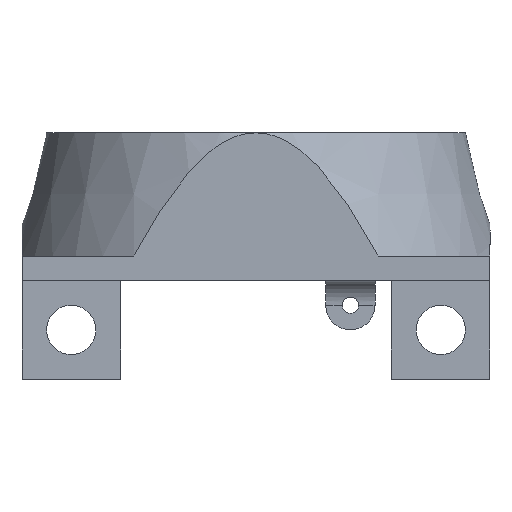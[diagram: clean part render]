
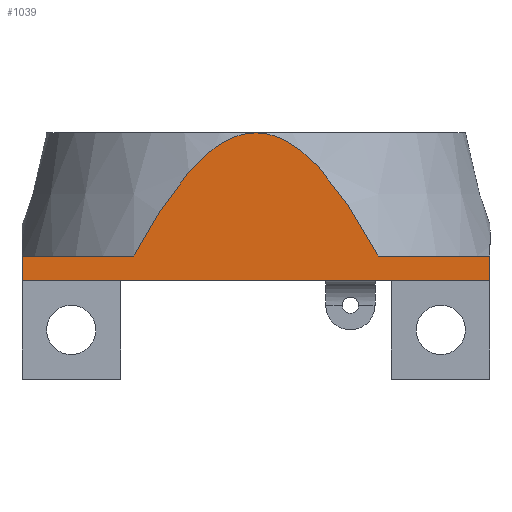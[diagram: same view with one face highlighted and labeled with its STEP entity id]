
A CAD part, left-side view. The second image highlights one B-rep face of the part: STEP entity #1039.
In plain terms, the highlighted planar face has unit normal (-1, 0, 0).
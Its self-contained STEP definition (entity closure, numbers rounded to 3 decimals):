
#65 = CARTESIAN_POINT ( 'NONE',  ( -24.047, 32.051, 2.538 ) ) ;
#81 = EDGE_CURVE ( 'NONE', #1986, #2008, #721, .T. ) ;
#107 = EDGE_CURVE ( 'NONE', #2039, #1986, #688, .T. ) ;
#151 = B_SPLINE_CURVE_WITH_KNOTS ( 'NONE', 3,
 ( #1533, #887, #882, #1527, #1524, #1520, #1516, #1514, #1508, #1505, #1500, #1493, #1483, #1474, #1468, #1466, #1463, #1462, #1455, #1453, #2058, #2047 ),
 .UNSPECIFIED., .F., .F.,
 ( 4, 2, 2, 2, 2, 2, 2, 2, 2, 2, 4 ),
 ( 0., 0.007, 0.01, 0.014, 0.017, 0.019, 0.021, 0.022, 0.024, 0.026, 0.027 ),
 .UNSPECIFIED. ) ;
#364 = DIRECTION ( 'NONE',  ( 0., -1., 0. ) ) ;
#367 = DIRECTION ( 'NONE',  ( 0., 0., -1. ) ) ;
#370 = CARTESIAN_POINT ( 'NONE',  ( -24.047, -0.893, 6.288 ) ) ;
#374 = CARTESIAN_POINT ( 'NONE',  ( -24.047, -39.199, 25.038 ) ) ;
#476 = CARTESIAN_POINT ( 'NONE',  ( -24.047, -39.199, 2.538 ) ) ;
#583 = CARTESIAN_POINT ( 'NONE',  ( -24.047, 32.051, 6.288 ) ) ;
#591 = CARTESIAN_POINT ( 'NONE',  ( -24.047, 15.015, 6.288 ) ) ;
#593 = CARTESIAN_POINT ( 'NONE',  ( -24.047, 13.938, 8.312 ) ) ;
#595 = CARTESIAN_POINT ( 'NONE',  ( -24.047, 12.81, 10.307 ) ) ;
#598 = CARTESIAN_POINT ( 'NONE',  ( -24.047, 10.991, 13.224 ) ) ;
#600 = CARTESIAN_POINT ( 'NONE',  ( -24.047, 10.363, 14.185 ) ) ;
#608 = CARTESIAN_POINT ( 'NONE',  ( -24.047, 9.056, 16.061 ) ) ;
#614 = CARTESIAN_POINT ( 'NONE',  ( -24.047, 8.377, 16.978 ) ) ;
#615 = CARTESIAN_POINT ( 'NONE',  ( -24.047, 6.947, 18.751 ) ) ;
#619 = CARTESIAN_POINT ( 'NONE',  ( -24.047, 6.198, 19.608 ) ) ;
#620 = CARTESIAN_POINT ( 'NONE',  ( -24.047, 4.993, 20.825 ) ) ;
#622 = CARTESIAN_POINT ( 'NONE',  ( -24.047, 4.578, 21.22 ) ) ;
#623 = CARTESIAN_POINT ( 'NONE',  ( -24.047, 3.713, 21.98 ) ) ;
#625 = CARTESIAN_POINT ( 'NONE',  ( -24.047, 3.262, 22.346 ) ) ;
#629 = CARTESIAN_POINT ( 'NONE',  ( -24.047, 1.868, 23.365 ) ) ;
#633 = CARTESIAN_POINT ( 'NONE',  ( -24.047, 0.881, 23.949 ) ) ;
#637 = CARTESIAN_POINT ( 'NONE',  ( -24.047, -1.284, 24.799 ) ) ;
#644 = CARTESIAN_POINT ( 'NONE',  ( -24.047, -3.574, 25.038 ) ) ;
#656 = CARTESIAN_POINT ( 'NONE',  ( -24.047, -2.406, 25.038 ) ) ;
#688 = LINE ( 'NONE', #1654, #696 ) ;
#694 = VECTOR ( 'NONE', #367, 1000. ) ;
#696 = VECTOR ( 'NONE', #1174, 1000. ) ;
#703 = VECTOR ( 'NONE', #364, 1000. ) ;
#710 = VECTOR ( 'NONE', #1718, 1000. ) ;
#714 = LINE ( 'NONE', #370, #703 ) ;
#721 = LINE ( 'NONE', #65, #710 ) ;
#743 = LINE ( 'NONE', #374, #694 ) ;
#747 = CARTESIAN_POINT ( 'NONE',  ( -24.047, 32.051, 2.538 ) ) ;
#825 = CARTESIAN_POINT ( 'NONE',  ( -24.047, 15.015, 6.288 ) ) ;
#849 = EDGE_CURVE ( 'NONE', #2095, #2044, #151, .T. ) ;
#882 = CARTESIAN_POINT ( 'NONE',  ( -24.047, -19.958, 10.305 ) ) ;
#887 = CARTESIAN_POINT ( 'NONE',  ( -24.047, -21.085, 8.312 ) ) ;
#1039 = ADVANCED_FACE ( 'NONE', ( #1063 ), #1399, .F. ) ;
#1063 = FACE_OUTER_BOUND ( 'NONE', #1076, .T. ) ;
#1068 = EDGE_CURVE ( 'NONE', #2095, #2137, #1089, .T. ) ;
#1076 = EDGE_LOOP ( 'NONE', ( #1779, #1772, #1704, #2197, #2210, #1501, #1831 ) ) ;
#1083 = VECTOR ( 'NONE', #1118, 1000. ) ;
#1089 = LINE ( 'NONE', #1121, #1083 ) ;
#1118 = DIRECTION ( 'NONE',  ( 0., -1., 0. ) ) ;
#1121 = CARTESIAN_POINT ( 'NONE',  ( -24.047, -0.893, 6.288 ) ) ;
#1146 = DIRECTION ( 'NONE',  ( 0., 0., -1. ) ) ;
#1149 = DIRECTION ( 'NONE',  ( 1., 0., 0. ) ) ;
#1152 = CARTESIAN_POINT ( 'NONE',  ( -24.047, 32.051, 25.038 ) ) ;
#1174 = DIRECTION ( 'NONE',  ( 0., 0., -1. ) ) ;
#1316 = EDGE_CURVE ( 'NONE', #2044, #2071, #2063, .T. ) ;
#1399 = PLANE ( 'NONE',  #1947 ) ;
#1436 = EDGE_CURVE ( 'NONE', #2137, #2008, #743, .T. ) ;
#1453 = CARTESIAN_POINT ( 'NONE',  ( -24.047, -4.733, 24.978 ) ) ;
#1455 = CARTESIAN_POINT ( 'NONE',  ( -24.047, -5.857, 24.751 ) ) ;
#1458 = EDGE_CURVE ( 'NONE', #2039, #2071, #714, .T. ) ;
#1462 = CARTESIAN_POINT ( 'NONE',  ( -24.047, -6.404, 24.586 ) ) ;
#1463 = CARTESIAN_POINT ( 'NONE',  ( -24.047, -7.473, 24.167 ) ) ;
#1466 = CARTESIAN_POINT ( 'NONE',  ( -24.047, -7.996, 23.913 ) ) ;
#1468 = CARTESIAN_POINT ( 'NONE',  ( -24.047, -8.991, 23.346 ) ) ;
#1474 = CARTESIAN_POINT ( 'NONE',  ( -24.047, -9.469, 23.032 ) ) ;
#1483 = CARTESIAN_POINT ( 'NONE',  ( -24.047, -10.393, 22.358 ) ) ;
#1493 = CARTESIAN_POINT ( 'NONE',  ( -24.047, -10.839, 21.997 ) ) ;
#1500 = CARTESIAN_POINT ( 'NONE',  ( -24.047, -11.705, 21.238 ) ) ;
#1501 = ORIENTED_EDGE ( 'NONE', *, *, #1436, .F. ) ;
#1505 = CARTESIAN_POINT ( 'NONE',  ( -24.047, -12.121, 20.843 ) ) ;
#1508 = CARTESIAN_POINT ( 'NONE',  ( -24.047, -13.33, 19.624 ) ) ;
#1514 = CARTESIAN_POINT ( 'NONE',  ( -24.047, -14.084, 18.763 ) ) ;
#1516 = CARTESIAN_POINT ( 'NONE',  ( -24.047, -15.523, 16.979 ) ) ;
#1520 = CARTESIAN_POINT ( 'NONE',  ( -24.047, -16.207, 16.055 ) ) ;
#1524 = CARTESIAN_POINT ( 'NONE',  ( -24.047, -17.516, 14.175 ) ) ;
#1527 = CARTESIAN_POINT ( 'NONE',  ( -24.047, -18.143, 13.217 ) ) ;
#1533 = CARTESIAN_POINT ( 'NONE',  ( -24.047, -22.162, 6.288 ) ) ;
#1654 = CARTESIAN_POINT ( 'NONE',  ( -24.047, 32.051, 25.038 ) ) ;
#1704 = ORIENTED_EDGE ( 'NONE', *, *, #1458, .F. ) ;
#1718 = DIRECTION ( 'NONE',  ( 0., -1., 0. ) ) ;
#1772 = ORIENTED_EDGE ( 'NONE', *, *, #1316, .T. ) ;
#1779 = ORIENTED_EDGE ( 'NONE', *, *, #849, .T. ) ;
#1831 = ORIENTED_EDGE ( 'NONE', *, *, #1068, .F. ) ;
#1947 = AXIS2_PLACEMENT_3D ( 'NONE', #1152, #1149, #1146 ) ;
#1986 = VERTEX_POINT ( 'NONE', #747 ) ;
#2008 = VERTEX_POINT ( 'NONE', #476 ) ;
#2039 = VERTEX_POINT ( 'NONE', #583 ) ;
#2044 = VERTEX_POINT ( 'NONE', #2376 ) ;
#2047 = CARTESIAN_POINT ( 'NONE',  ( -24.047, -3.574, 25.038 ) ) ;
#2058 = CARTESIAN_POINT ( 'NONE',  ( -24.047, -4.153, 25.038 ) ) ;
#2063 = B_SPLINE_CURVE_WITH_KNOTS ( 'NONE', 3,
 ( #644, #656, #637, #633, #629, #625, #623, #622, #620, #619, #615, #614, #608, #600, #598, #595, #593, #591 ),
 .UNSPECIFIED., .F., .F.,
 ( 4, 2, 2, 2, 2, 2, 2, 2, 4 ),
 ( 0., 0.003, 0.007, 0.009, 0.01, 0.014, 0.017, 0.021, 0.027 ),
 .UNSPECIFIED. ) ;
#2071 = VERTEX_POINT ( 'NONE', #825 ) ;
#2095 = VERTEX_POINT ( 'NONE', #2224 ) ;
#2137 = VERTEX_POINT ( 'NONE', #2281 ) ;
#2197 = ORIENTED_EDGE ( 'NONE', *, *, #107, .T. ) ;
#2210 = ORIENTED_EDGE ( 'NONE', *, *, #81, .T. ) ;
#2224 = CARTESIAN_POINT ( 'NONE',  ( -24.047, -22.162, 6.288 ) ) ;
#2281 = CARTESIAN_POINT ( 'NONE',  ( -24.047, -39.199, 6.288 ) ) ;
#2376 = CARTESIAN_POINT ( 'NONE',  ( -24.047, -3.574, 25.038 ) ) ;
